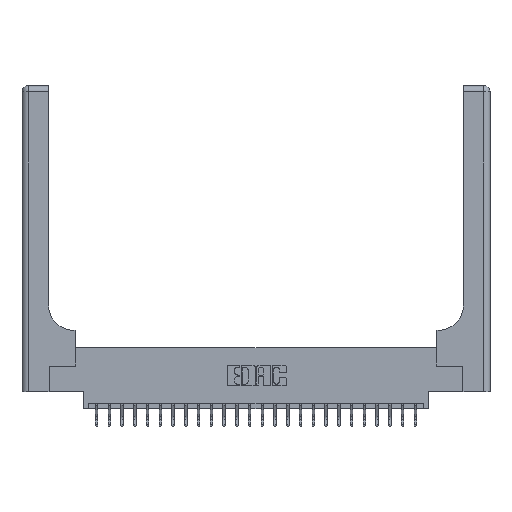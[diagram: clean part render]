
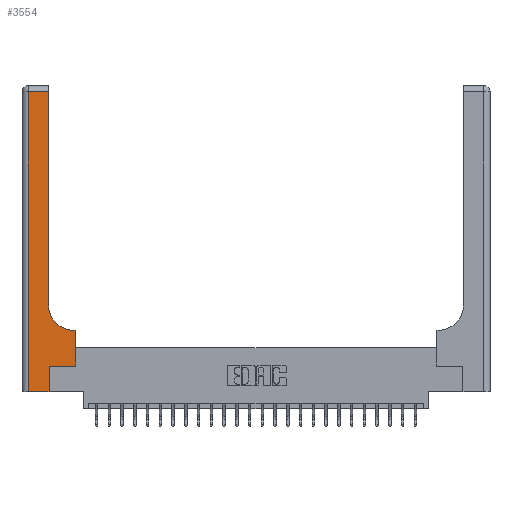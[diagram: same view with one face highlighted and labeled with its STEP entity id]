
A CAD part, top view. The second image highlights one B-rep face of the part: STEP entity #3554.
In plain terms, the highlighted planar face has unit normal (0, 0, 1).
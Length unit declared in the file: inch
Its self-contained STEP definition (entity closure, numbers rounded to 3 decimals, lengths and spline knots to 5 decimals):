
#150 = LINE ( 'NONE', #21120, #13422 ) ;
#910 = VERTEX_POINT ( 'NONE', #6788 ) ;
#1243 = LINE ( 'NONE', #9028, #8484 ) ;
#1452 = DIRECTION ( 'NONE',  ( 0., 1., 0. ) ) ;
#1500 = CARTESIAN_POINT ( 'NONE',  ( 0.06, 0., 0.37 ) ) ;
#1820 = EDGE_CURVE ( 'NONE', #24254, #2764, #12795, .T. ) ;
#1905 = CARTESIAN_POINT ( 'NONE',  ( 0.265, 0., 0.37 ) ) ;
#2508 = ORIENTED_EDGE ( 'NONE', *, *, #20041, .T. ) ;
#2764 = VERTEX_POINT ( 'NONE', #9025 ) ;
#3229 = PLANE ( 'NONE',  #20105 ) ;
#3396 = ORIENTED_EDGE ( 'NONE', *, *, #21793, .T. ) ;
#3554 = ADVANCED_FACE ( 'NONE', ( #24568 ), #3229, .F. ) ;
#3677 = DIRECTION ( 'NONE',  ( -1., 0., 0. ) ) ;
#3930 = VECTOR ( 'NONE', #1452, 39.37008 ) ;
#4609 = EDGE_CURVE ( 'NONE', #4809, #12240, #4773, .T. ) ;
#4773 = LINE ( 'NONE', #12529, #24462 ) ;
#4809 = VERTEX_POINT ( 'NONE', #15910 ) ;
#4851 = ORIENTED_EDGE ( 'NONE', *, *, #9618, .T. ) ;
#5369 = CARTESIAN_POINT ( 'NONE',  ( 0.528, 0.25, 0.37 ) ) ;
#5695 = EDGE_CURVE ( 'NONE', #11438, #12400, #6205, .T. ) ;
#6205 = LINE ( 'NONE', #11812, #22494 ) ;
#6363 = LINE ( 'NONE', #1905, #24157 ) ;
#6788 = CARTESIAN_POINT ( 'NONE',  ( 0.51, 0.6, 0.37 ) ) ;
#7174 = CARTESIAN_POINT ( 'NONE',  ( 0., 3., 0.37 ) ) ;
#7723 = CARTESIAN_POINT ( 'NONE',  ( 0.06, 2.94, 0.37 ) ) ;
#8032 = CARTESIAN_POINT ( 'NONE',  ( 0.265, 0., 0.37 ) ) ;
#8442 = DIRECTION ( 'NONE',  ( 1., 0., 0. ) ) ;
#8484 = VECTOR ( 'NONE', #18296, 39.37008 ) ;
#8691 = CARTESIAN_POINT ( 'NONE',  ( 0.51, 0.85, 0.37 ) ) ;
#9025 = CARTESIAN_POINT ( 'NONE',  ( 0.26, 2.94, 0.37 ) ) ;
#9028 = CARTESIAN_POINT ( 'NONE',  ( 0., 0., 0.37 ) ) ;
#9618 = EDGE_CURVE ( 'NONE', #20904, #4809, #6363, .T. ) ;
#9734 = DIRECTION ( 'NONE',  ( -1., 0., 0. ) ) ;
#9735 = ORIENTED_EDGE ( 'NONE', *, *, #1820, .T. ) ;
#9890 = CIRCLE ( 'NONE', #16346, 0.25 ) ;
#10036 = DIRECTION ( 'NONE',  ( 0., -1., 0. ) ) ;
#10272 = ORIENTED_EDGE ( 'NONE', *, *, #21954, .T. ) ;
#10874 = DIRECTION ( 'NONE',  ( 0., 0., -1. ) ) ;
#11071 = CARTESIAN_POINT ( 'NONE',  ( 0.528, 0.25, 0.37 ) ) ;
#11099 = DIRECTION ( 'NONE',  ( 0., 1., 0. ) ) ;
#11222 = LINE ( 'NONE', #5369, #18021 ) ;
#11438 = VERTEX_POINT ( 'NONE', #7723 ) ;
#11560 = VERTEX_POINT ( 'NONE', #19621 ) ;
#11812 = CARTESIAN_POINT ( 'NONE',  ( 0.06, 3., 0.37 ) ) ;
#12240 = VERTEX_POINT ( 'NONE', #11071 ) ;
#12400 = VERTEX_POINT ( 'NONE', #1500 ) ;
#12529 = CARTESIAN_POINT ( 'NONE',  ( 0.265, 0.25, 0.37 ) ) ;
#12795 = LINE ( 'NONE', #13297, #3930 ) ;
#13079 = ORIENTED_EDGE ( 'NONE', *, *, #13709, .T. ) ;
#13297 = CARTESIAN_POINT ( 'NONE',  ( 0.26, 3., 0.37 ) ) ;
#13422 = VECTOR ( 'NONE', #9734, 39.37008 ) ;
#13709 = EDGE_CURVE ( 'NONE', #12400, #20904, #1243, .T. ) ;
#14676 = DIRECTION ( 'NONE',  ( 1., 0., 0. ) ) ;
#15910 = CARTESIAN_POINT ( 'NONE',  ( 0.265, 0.25, 0.37 ) ) ;
#16240 = ORIENTED_EDGE ( 'NONE', *, *, #5695, .T. ) ;
#16346 = AXIS2_PLACEMENT_3D ( 'NONE', #8691, #19850, #8442 ) ;
#17132 = VECTOR ( 'NONE', #3677, 39.37008 ) ;
#17563 = EDGE_CURVE ( 'NONE', #11560, #910, #150, .T. ) ;
#18021 = VECTOR ( 'NONE', #11099, 39.37008 ) ;
#18296 = DIRECTION ( 'NONE',  ( 1., 0., 0. ) ) ;
#18451 = ORIENTED_EDGE ( 'NONE', *, *, #17563, .T. ) ;
#18601 = DIRECTION ( 'NONE',  ( -1., 0., 0. ) ) ;
#19153 = CARTESIAN_POINT ( 'NONE',  ( 0., 2.94, 0.37 ) ) ;
#19155 = DIRECTION ( 'NONE',  ( 0., 1., 0. ) ) ;
#19173 = ORIENTED_EDGE ( 'NONE', *, *, #4609, .T. ) ;
#19621 = CARTESIAN_POINT ( 'NONE',  ( 0.528, 0.6, 0.37 ) ) ;
#19760 = CARTESIAN_POINT ( 'NONE',  ( 0.26, 0.85, 0.37 ) ) ;
#19850 = DIRECTION ( 'NONE',  ( 0., 0., -1. ) ) ;
#20041 = EDGE_CURVE ( 'NONE', #2764, #11438, #21058, .T. ) ;
#20105 = AXIS2_PLACEMENT_3D ( 'NONE', #7174, #10874, #18601 ) ;
#20904 = VERTEX_POINT ( 'NONE', #8032 ) ;
#21058 = LINE ( 'NONE', #19153, #17132 ) ;
#21120 = CARTESIAN_POINT ( 'NONE',  ( 0.26, 0.6, 0.37 ) ) ;
#21793 = EDGE_CURVE ( 'NONE', #910, #24254, #9890, .T. ) ;
#21954 = EDGE_CURVE ( 'NONE', #12240, #11560, #11222, .T. ) ;
#22446 = EDGE_LOOP ( 'NONE', ( #9735, #2508, #16240, #13079, #4851, #19173, #10272, #18451, #3396 ) ) ;
#22494 = VECTOR ( 'NONE', #10036, 39.37008 ) ;
#24157 = VECTOR ( 'NONE', #19155, 39.37008 ) ;
#24254 = VERTEX_POINT ( 'NONE', #19760 ) ;
#24462 = VECTOR ( 'NONE', #14676, 39.37008 ) ;
#24568 = FACE_OUTER_BOUND ( 'NONE', #22446, .T. ) ;
